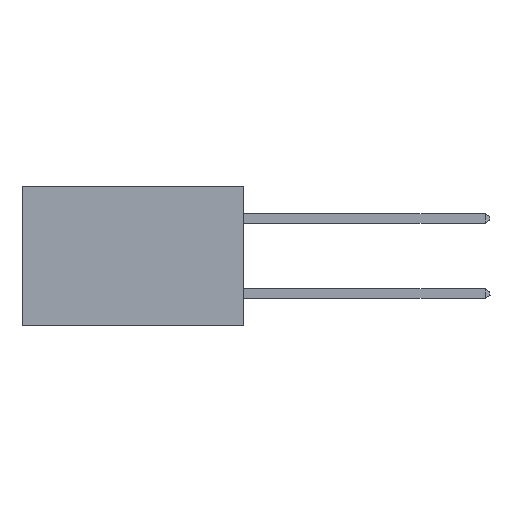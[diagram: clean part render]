
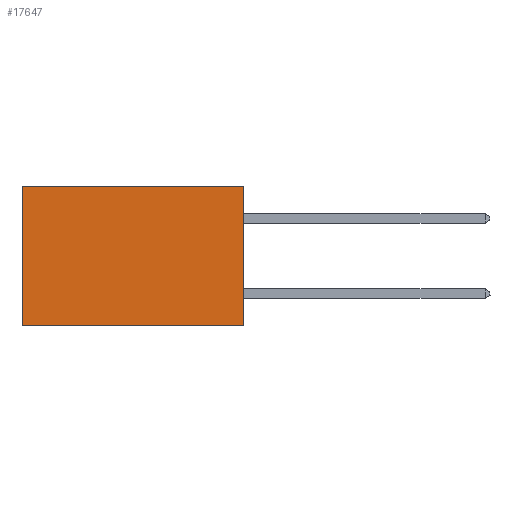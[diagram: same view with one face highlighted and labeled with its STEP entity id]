
A CAD part, left-side view. The second image highlights one B-rep face of the part: STEP entity #17647.
In plain terms, the highlighted planar face has unit normal (-1, 0, 0).
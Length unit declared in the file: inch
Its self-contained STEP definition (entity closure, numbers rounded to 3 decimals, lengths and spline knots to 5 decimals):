
#47 = CARTESIAN_POINT ( 'NONE',  ( 0.277, 0.59, -0.37 ) ) ;
#501 = LINE ( 'NONE', #8428, #13939 ) ;
#984 = VECTOR ( 'NONE', #21571, 39.37008 ) ;
#1309 = VECTOR ( 'NONE', #19651, 39.37008 ) ;
#3198 = AXIS2_PLACEMENT_3D ( 'NONE', #9935, #8250, #20352 ) ;
#4179 = EDGE_CURVE ( 'NONE', #4505, #17865, #5688, .T. ) ;
#4505 = VERTEX_POINT ( 'NONE', #15667 ) ;
#5391 = EDGE_CURVE ( 'NONE', #19744, #17865, #9701, .T. ) ;
#5688 = LINE ( 'NONE', #14750, #984 ) ;
#5840 = CARTESIAN_POINT ( 'NONE',  ( 0.277, 0.59, -0.37 ) ) ;
#6478 = PLANE ( 'NONE',  #3198 ) ;
#6606 = DIRECTION ( 'NONE',  ( 0., 0., -1. ) ) ;
#8216 = ORIENTED_EDGE ( 'NONE', *, *, #16337, .F. ) ;
#8250 = DIRECTION ( 'NONE',  ( 1., 0., 0. ) ) ;
#8428 = CARTESIAN_POINT ( 'NONE',  ( 0.277, 0., 0. ) ) ;
#9701 = LINE ( 'NONE', #5840, #13753 ) ;
#9935 = CARTESIAN_POINT ( 'NONE',  ( 0.277, 0., -0.37 ) ) ;
#10177 = DIRECTION ( 'NONE',  ( 0., 1., 0. ) ) ;
#10379 = VERTEX_POINT ( 'NONE', #16316 ) ;
#10630 = ORIENTED_EDGE ( 'NONE', *, *, #4179, .F. ) ;
#11698 = ORIENTED_EDGE ( 'NONE', *, *, #21469, .T. ) ;
#13043 = EDGE_LOOP ( 'NONE', ( #18740, #10630, #8216, #11698 ) ) ;
#13753 = VECTOR ( 'NONE', #6606, 39.37008 ) ;
#13939 = VECTOR ( 'NONE', #10177, 39.37008 ) ;
#14750 = CARTESIAN_POINT ( 'NONE',  ( 0.277, 0., -0.37 ) ) ;
#15295 = LINE ( 'NONE', #17919, #1309 ) ;
#15605 = CARTESIAN_POINT ( 'NONE',  ( 0.277, 0.59, 0. ) ) ;
#15667 = CARTESIAN_POINT ( 'NONE',  ( 0.277, 0., -0.37 ) ) ;
#16316 = CARTESIAN_POINT ( 'NONE',  ( 0.277, 0., 0. ) ) ;
#16337 = EDGE_CURVE ( 'NONE', #10379, #4505, #15295, .T. ) ;
#17647 = ADVANCED_FACE ( 'NONE', ( #19241 ), #6478, .F. ) ;
#17865 = VERTEX_POINT ( 'NONE', #47 ) ;
#17919 = CARTESIAN_POINT ( 'NONE',  ( 0.277, 0., -0.37 ) ) ;
#18740 = ORIENTED_EDGE ( 'NONE', *, *, #5391, .T. ) ;
#19241 = FACE_OUTER_BOUND ( 'NONE', #13043, .T. ) ;
#19651 = DIRECTION ( 'NONE',  ( 0., 0., -1. ) ) ;
#19744 = VERTEX_POINT ( 'NONE', #15605 ) ;
#20352 = DIRECTION ( 'NONE',  ( 0., 0., -1. ) ) ;
#21469 = EDGE_CURVE ( 'NONE', #10379, #19744, #501, .T. ) ;
#21571 = DIRECTION ( 'NONE',  ( 0., 1., 0. ) ) ;
